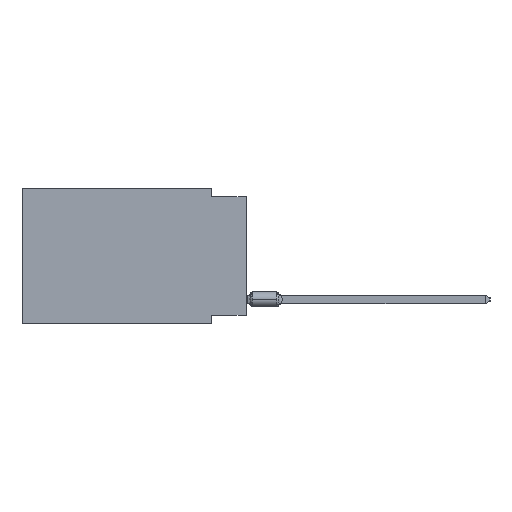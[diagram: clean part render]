
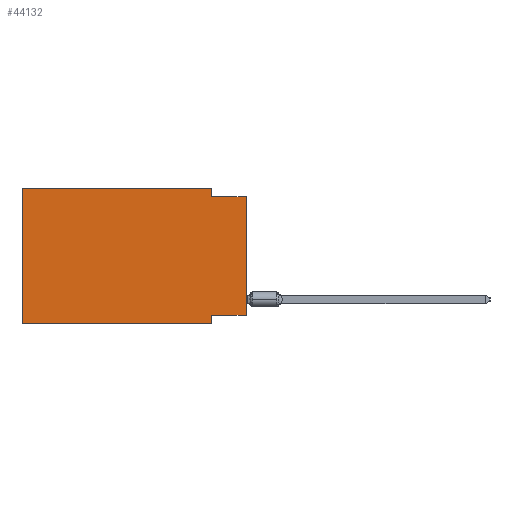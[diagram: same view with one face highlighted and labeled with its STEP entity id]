
A CAD part, left-side view. The second image highlights one B-rep face of the part: STEP entity #44132.
In plain terms, the highlighted planar face has unit normal (-1, 0, 0).
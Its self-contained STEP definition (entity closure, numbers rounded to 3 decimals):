
#2883 = LINE ( 'NONE', #25868, #47134 ) ;
#2971 = CARTESIAN_POINT ( 'NONE',  ( 0., 16.383, 0. ) ) ;
#4256 = CARTESIAN_POINT ( 'NONE',  ( 0., 0., -9.271 ) ) ;
#4321 = VERTEX_POINT ( 'NONE', #43403 ) ;
#6513 = CARTESIAN_POINT ( 'NONE',  ( 0., 16.383, -9.906 ) ) ;
#6907 = CARTESIAN_POINT ( 'NONE',  ( 0., 2.54, -0.635 ) ) ;
#11854 = VERTEX_POINT ( 'NONE', #28552 ) ;
#13048 = VERTEX_POINT ( 'NONE', #45100 ) ;
#13545 = DIRECTION ( 'NONE',  ( 0., 0., -1. ) ) ;
#14446 = LINE ( 'NONE', #42665, #37407 ) ;
#14577 = EDGE_CURVE ( 'NONE', #17711, #13048, #37124, .T. ) ;
#15190 = LINE ( 'NONE', #4256, #26432 ) ;
#16817 = VECTOR ( 'NONE', #25375, 1000. ) ;
#17711 = VERTEX_POINT ( 'NONE', #6907 ) ;
#17915 = CARTESIAN_POINT ( 'NONE',  ( 0., 16.383, -9.906 ) ) ;
#19815 = DIRECTION ( 'NONE',  ( 0., -1., 0. ) ) ;
#21039 = ORIENTED_EDGE ( 'NONE', *, *, #51969, .F. ) ;
#21978 = LINE ( 'NONE', #56243, #48626 ) ;
#25375 = DIRECTION ( 'NONE',  ( 0., 0., -1. ) ) ;
#25868 = CARTESIAN_POINT ( 'NONE',  ( 0., 2.54, 0. ) ) ;
#26432 = VECTOR ( 'NONE', #60728, 1000. ) ;
#28552 = CARTESIAN_POINT ( 'NONE',  ( 0., 2.54, 0. ) ) ;
#28750 = LINE ( 'NONE', #74270, #42945 ) ;
#29579 = DIRECTION ( 'NONE',  ( 0., -1., 0. ) ) ;
#30282 = CARTESIAN_POINT ( 'NONE',  ( 0., 2.54, -9.906 ) ) ;
#32865 = EDGE_CURVE ( 'NONE', #69803, #33419, #52867, .T. ) ;
#33011 = EDGE_CURVE ( 'NONE', #65464, #69803, #15190, .T. ) ;
#33419 = VERTEX_POINT ( 'NONE', #65962 ) ;
#34568 = EDGE_LOOP ( 'NONE', ( #73575, #45007, #54373, #46170, #21039, #38601, #35569, #66965 ) ) ;
#35422 = VECTOR ( 'NONE', #29579, 1000. ) ;
#35569 = ORIENTED_EDGE ( 'NONE', *, *, #32865, .F. ) ;
#36497 = PLANE ( 'NONE',  #45993 ) ;
#37124 = LINE ( 'NONE', #60822, #64675 ) ;
#37241 = DIRECTION ( 'NONE',  ( 1., 0., 0. ) ) ;
#37407 = VECTOR ( 'NONE', #65635, 1000. ) ;
#38601 = ORIENTED_EDGE ( 'NONE', *, *, #47617, .T. ) ;
#42093 = EDGE_CURVE ( 'NONE', #4321, #11854, #14446, .T. ) ;
#42665 = CARTESIAN_POINT ( 'NONE',  ( 0., 16.383, 0. ) ) ;
#42945 = VECTOR ( 'NONE', #46044, 1000. ) ;
#43403 = CARTESIAN_POINT ( 'NONE',  ( 0., 16.383, 0. ) ) ;
#44132 = ADVANCED_FACE ( 'NONE', ( #54927 ), #36497, .F. ) ;
#44639 = EDGE_CURVE ( 'NONE', #11854, #17711, #2883, .T. ) ;
#45007 = ORIENTED_EDGE ( 'NONE', *, *, #14577, .F. ) ;
#45100 = CARTESIAN_POINT ( 'NONE',  ( 0., 0., -0.635 ) ) ;
#45841 = CARTESIAN_POINT ( 'NONE',  ( 0., 0., -9.271 ) ) ;
#45993 = AXIS2_PLACEMENT_3D ( 'NONE', #2971, #37241, #13545 ) ;
#46044 = DIRECTION ( 'NONE',  ( 0., 0., 1. ) ) ;
#46170 = ORIENTED_EDGE ( 'NONE', *, *, #42093, .F. ) ;
#47134 = VECTOR ( 'NONE', #50575, 1000. ) ;
#47617 = EDGE_CURVE ( 'NONE', #64662, #33419, #69458, .T. ) ;
#47771 = EDGE_CURVE ( 'NONE', #65464, #13048, #21978, .T. ) ;
#48626 = VECTOR ( 'NONE', #67872, 1000. ) ;
#50575 = DIRECTION ( 'NONE',  ( 0., 0., -1. ) ) ;
#51969 = EDGE_CURVE ( 'NONE', #64662, #4321, #28750, .T. ) ;
#52867 = LINE ( 'NONE', #30282, #16817 ) ;
#54373 = ORIENTED_EDGE ( 'NONE', *, *, #44639, .F. ) ;
#54927 = FACE_OUTER_BOUND ( 'NONE', #34568, .T. ) ;
#56243 = CARTESIAN_POINT ( 'NONE',  ( 0., 0., 0. ) ) ;
#60728 = DIRECTION ( 'NONE',  ( 0., 1., 0. ) ) ;
#60822 = CARTESIAN_POINT ( 'NONE',  ( 0., 0., -0.635 ) ) ;
#64662 = VERTEX_POINT ( 'NONE', #6513 ) ;
#64675 = VECTOR ( 'NONE', #19815, 1000. ) ;
#65464 = VERTEX_POINT ( 'NONE', #45841 ) ;
#65635 = DIRECTION ( 'NONE',  ( 0., -1., 0. ) ) ;
#65962 = CARTESIAN_POINT ( 'NONE',  ( 0., 2.54, -9.906 ) ) ;
#66965 = ORIENTED_EDGE ( 'NONE', *, *, #33011, .F. ) ;
#67872 = DIRECTION ( 'NONE',  ( 0., 0., 1. ) ) ;
#69458 = LINE ( 'NONE', #17915, #35422 ) ;
#69803 = VERTEX_POINT ( 'NONE', #71566 ) ;
#71566 = CARTESIAN_POINT ( 'NONE',  ( 0., 2.54, -9.271 ) ) ;
#73575 = ORIENTED_EDGE ( 'NONE', *, *, #47771, .T. ) ;
#74270 = CARTESIAN_POINT ( 'NONE',  ( 0., 16.383, 0. ) ) ;
